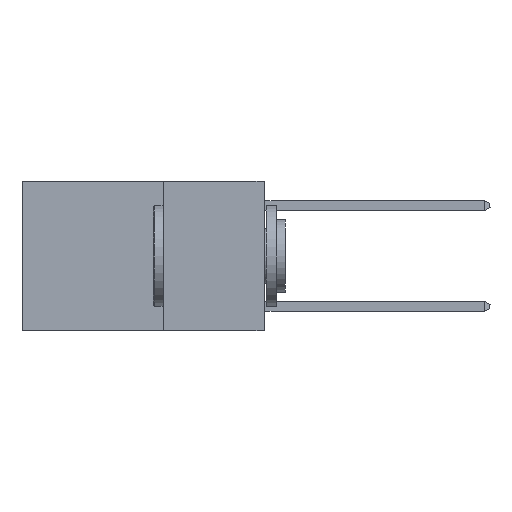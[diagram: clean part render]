
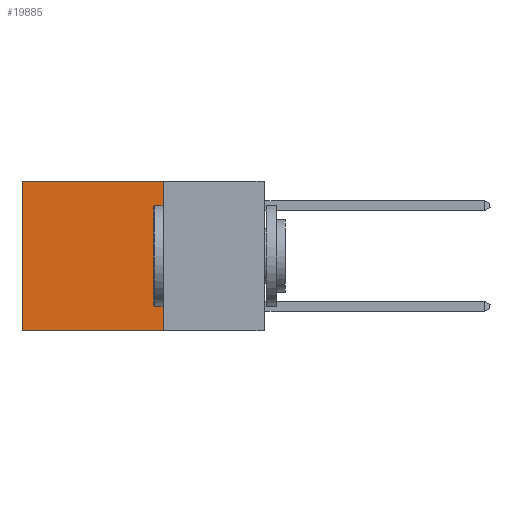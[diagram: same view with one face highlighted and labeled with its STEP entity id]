
A CAD part, left-side view. The second image highlights one B-rep face of the part: STEP entity #19885.
In plain terms, the highlighted planar face has unit normal (-1, 0, 0).
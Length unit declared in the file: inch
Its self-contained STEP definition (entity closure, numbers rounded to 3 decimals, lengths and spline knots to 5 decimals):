
#126 = LINE ( 'NONE', #11487, #656 ) ;
#656 = VECTOR ( 'NONE', #18213, 39.37008 ) ;
#1001 = DIRECTION ( 'NONE',  ( 0., 0., -1. ) ) ;
#1011 = CARTESIAN_POINT ( 'NONE',  ( 0.2625, 0.6, -0.37 ) ) ;
#1575 = LINE ( 'NONE', #21748, #4109 ) ;
#1732 = LINE ( 'NONE', #29276, #23878 ) ;
#3722 = DIRECTION ( 'NONE',  ( 0., 0., -1. ) ) ;
#4109 = VECTOR ( 'NONE', #17408, 39.37008 ) ;
#5619 = FACE_OUTER_BOUND ( 'NONE', #22510, .T. ) ;
#5812 = ORIENTED_EDGE ( 'NONE', *, *, #19750, .F. ) ;
#8566 = EDGE_CURVE ( 'NONE', #19019, #27797, #1575, .T. ) ;
#9481 = VERTEX_POINT ( 'NONE', #23798 ) ;
#11487 = CARTESIAN_POINT ( 'NONE',  ( 0.2625, 0.25, -0.37 ) ) ;
#12699 = CARTESIAN_POINT ( 'NONE',  ( 0.2625, 0.6, 0. ) ) ;
#13434 = EDGE_CURVE ( 'NONE', #27797, #22577, #1732, .T. ) ;
#13524 = DIRECTION ( 'NONE',  ( 0., 0., -1. ) ) ;
#14748 = ORIENTED_EDGE ( 'NONE', *, *, #13434, .T. ) ;
#14917 = LINE ( 'NONE', #24217, #25202 ) ;
#15290 = ORIENTED_EDGE ( 'NONE', *, *, #28103, .F. ) ;
#17408 = DIRECTION ( 'NONE',  ( 0., 1., 0. ) ) ;
#17988 = ORIENTED_EDGE ( 'NONE', *, *, #8566, .T. ) ;
#18213 = DIRECTION ( 'NONE',  ( 0., 1., 0. ) ) ;
#19019 = VERTEX_POINT ( 'NONE', #27448 ) ;
#19086 = CARTESIAN_POINT ( 'NONE',  ( 0.2625, 0.25, 0. ) ) ;
#19750 = EDGE_CURVE ( 'NONE', #9481, #22577, #126, .T. ) ;
#19885 = ADVANCED_FACE ( 'NONE', ( #5619 ), #28099, .F. ) ;
#21748 = CARTESIAN_POINT ( 'NONE',  ( 0.2625, 0.25, 0. ) ) ;
#22510 = EDGE_LOOP ( 'NONE', ( #14748, #5812, #15290, #17988 ) ) ;
#22577 = VERTEX_POINT ( 'NONE', #1011 ) ;
#23798 = CARTESIAN_POINT ( 'NONE',  ( 0.2625, 0.25, -0.37 ) ) ;
#23878 = VECTOR ( 'NONE', #13524, 39.37008 ) ;
#24217 = CARTESIAN_POINT ( 'NONE',  ( 0.2625, 0.25, 0. ) ) ;
#25202 = VECTOR ( 'NONE', #3722, 39.37008 ) ;
#25465 = AXIS2_PLACEMENT_3D ( 'NONE', #19086, #25856, #1001 ) ;
#25856 = DIRECTION ( 'NONE',  ( 1., 0., 0. ) ) ;
#27448 = CARTESIAN_POINT ( 'NONE',  ( 0.2625, 0.25, 0. ) ) ;
#27797 = VERTEX_POINT ( 'NONE', #12699 ) ;
#28099 = PLANE ( 'NONE',  #25465 ) ;
#28103 = EDGE_CURVE ( 'NONE', #19019, #9481, #14917, .T. ) ;
#29276 = CARTESIAN_POINT ( 'NONE',  ( 0.2625, 0.6, 0. ) ) ;
